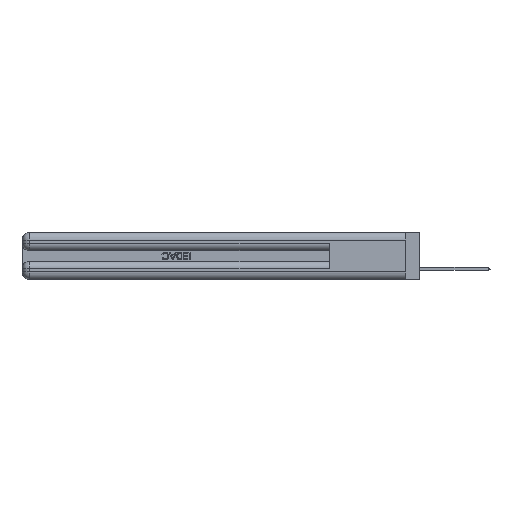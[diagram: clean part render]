
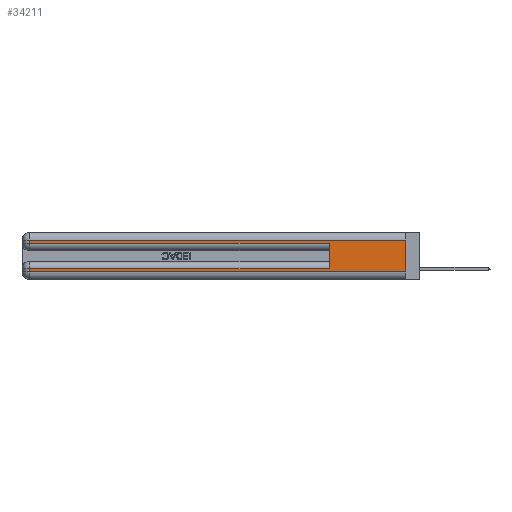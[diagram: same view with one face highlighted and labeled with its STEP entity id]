
A CAD part, left-side view. The second image highlights one B-rep face of the part: STEP entity #34211.
In plain terms, the highlighted planar face has unit normal (-1, 0, 0).
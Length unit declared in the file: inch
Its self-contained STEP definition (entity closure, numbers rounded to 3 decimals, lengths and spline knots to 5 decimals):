
#306 = LINE ( 'NONE', #16904, #36140 ) ;
#867 = LINE ( 'NONE', #39815, #18728 ) ;
#919 = VECTOR ( 'NONE', #3320, 39.37008 ) ;
#1488 = CARTESIAN_POINT ( 'NONE',  ( 0., 0., 0.285 ) ) ;
#1560 = CARTESIAN_POINT ( 'NONE',  ( 0., 0., 0.37 ) ) ;
#1707 = PLANE ( 'NONE',  #30695 ) ;
#3320 = DIRECTION ( 'NONE',  ( 0., 0., -1. ) ) ;
#3779 = VERTEX_POINT ( 'NONE', #34108 ) ;
#4612 = ORIENTED_EDGE ( 'NONE', *, *, #9556, .T. ) ;
#4931 = EDGE_CURVE ( 'NONE', #3779, #21198, #16940, .T. ) ;
#5001 = DIRECTION ( 'NONE',  ( 0., -1., 0. ) ) ;
#5275 = CARTESIAN_POINT ( 'NONE',  ( 0., 2.94, 0.37 ) ) ;
#5949 = CARTESIAN_POINT ( 'NONE',  ( 0., 0.6, 0.285 ) ) ;
#6099 = ORIENTED_EDGE ( 'NONE', *, *, #41169, .T. ) ;
#7029 = ORIENTED_EDGE ( 'NONE', *, *, #42457, .T. ) ;
#7392 = CARTESIAN_POINT ( 'NONE',  ( 0., 2.94, 0.37 ) ) ;
#8149 = DIRECTION ( 'NONE',  ( 0., 0., -1. ) ) ;
#9171 = FACE_OUTER_BOUND ( 'NONE', #28890, .T. ) ;
#9191 = LINE ( 'NONE', #44229, #33606 ) ;
#9556 = EDGE_CURVE ( 'NONE', #27646, #30161, #28112, .T. ) ;
#11006 = VERTEX_POINT ( 'NONE', #15800 ) ;
#11538 = DIRECTION ( 'NONE',  ( 0., -1., 0. ) ) ;
#12983 = CARTESIAN_POINT ( 'NONE',  ( 0., 2.94, 0.285 ) ) ;
#13062 = CARTESIAN_POINT ( 'NONE',  ( 0., 0., 0.06 ) ) ;
#13430 = VECTOR ( 'NONE', #11538, 39.37008 ) ;
#15262 = ORIENTED_EDGE ( 'NONE', *, *, #20927, .T. ) ;
#15800 = CARTESIAN_POINT ( 'NONE',  ( 0., 2.94, 0.31 ) ) ;
#16710 = VERTEX_POINT ( 'NONE', #40055 ) ;
#16904 = CARTESIAN_POINT ( 'NONE',  ( 0., 0., 0.37 ) ) ;
#16940 = LINE ( 'NONE', #44334, #19068 ) ;
#17345 = LINE ( 'NONE', #5275, #43962 ) ;
#17393 = EDGE_CURVE ( 'NONE', #16710, #11006, #867, .T. ) ;
#17433 = EDGE_CURVE ( 'NONE', #16710, #30161, #306, .T. ) ;
#18427 = LINE ( 'NONE', #1488, #22807 ) ;
#18728 = VECTOR ( 'NONE', #25668, 39.37008 ) ;
#19068 = VECTOR ( 'NONE', #43736, 39.37008 ) ;
#19881 = DIRECTION ( 'NONE',  ( 0., 1., 0. ) ) ;
#20765 = ORIENTED_EDGE ( 'NONE', *, *, #17393, .T. ) ;
#20927 = EDGE_CURVE ( 'NONE', #23551, #21198, #18427, .T. ) ;
#21198 = VERTEX_POINT ( 'NONE', #5949 ) ;
#22807 = VECTOR ( 'NONE', #5001, 39.37008 ) ;
#23551 = VERTEX_POINT ( 'NONE', #12983 ) ;
#25668 = DIRECTION ( 'NONE',  ( 0., 1., 0. ) ) ;
#25790 = CARTESIAN_POINT ( 'NONE',  ( 0., 2.94, 0.06 ) ) ;
#25825 = DIRECTION ( 'NONE',  ( 0., 0., -1. ) ) ;
#27646 = VERTEX_POINT ( 'NONE', #25790 ) ;
#28112 = LINE ( 'NONE', #32332, #13430 ) ;
#28890 = EDGE_LOOP ( 'NONE', ( #44126, #20765, #7029, #15262, #36419, #6099, #31206, #4612 ) ) ;
#28995 = VERTEX_POINT ( 'NONE', #40207 ) ;
#30161 = VERTEX_POINT ( 'NONE', #13062 ) ;
#30695 = AXIS2_PLACEMENT_3D ( 'NONE', #1560, #32819, #25825 ) ;
#31206 = ORIENTED_EDGE ( 'NONE', *, *, #40219, .T. ) ;
#32332 = CARTESIAN_POINT ( 'NONE',  ( 0., 0., 0.06 ) ) ;
#32819 = DIRECTION ( 'NONE',  ( 1., 0., 0. ) ) ;
#33606 = VECTOR ( 'NONE', #19881, 39.37008 ) ;
#34009 = LINE ( 'NONE', #7392, #919 ) ;
#34108 = CARTESIAN_POINT ( 'NONE',  ( 0., 0.6, 0.085 ) ) ;
#34211 = ADVANCED_FACE ( 'NONE', ( #9171 ), #1707, .F. ) ;
#36140 = VECTOR ( 'NONE', #44529, 39.37008 ) ;
#36419 = ORIENTED_EDGE ( 'NONE', *, *, #4931, .F. ) ;
#39815 = CARTESIAN_POINT ( 'NONE',  ( 0., 0., 0.31 ) ) ;
#40055 = CARTESIAN_POINT ( 'NONE',  ( 0., 0., 0.31 ) ) ;
#40207 = CARTESIAN_POINT ( 'NONE',  ( 0., 2.94, 0.085 ) ) ;
#40219 = EDGE_CURVE ( 'NONE', #28995, #27646, #17345, .T. ) ;
#41169 = EDGE_CURVE ( 'NONE', #3779, #28995, #9191, .T. ) ;
#42457 = EDGE_CURVE ( 'NONE', #11006, #23551, #34009, .T. ) ;
#43736 = DIRECTION ( 'NONE',  ( 0., 0., 1. ) ) ;
#43962 = VECTOR ( 'NONE', #8149, 39.37008 ) ;
#44126 = ORIENTED_EDGE ( 'NONE', *, *, #17433, .F. ) ;
#44229 = CARTESIAN_POINT ( 'NONE',  ( 0., 0., 0.085 ) ) ;
#44334 = CARTESIAN_POINT ( 'NONE',  ( 0., 0.6, 0.145 ) ) ;
#44529 = DIRECTION ( 'NONE',  ( 0., 0., -1. ) ) ;
